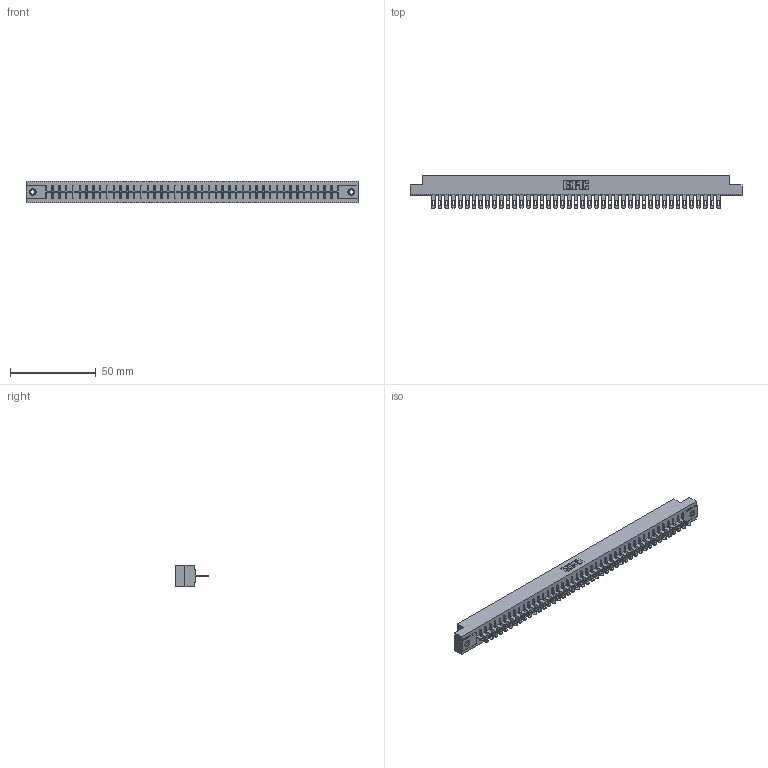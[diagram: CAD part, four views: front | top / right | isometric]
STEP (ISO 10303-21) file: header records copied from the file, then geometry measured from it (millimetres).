
FILE_DESCRIPTION (( 'STEP AP203' ), '1' );
FILE_NAME ('356-043-400-107.STEP', '2020-09-24T01:46:20', ( '' ), ( '' ), 'SwSTEP 2.0', 'SolidWorks 2020', '' );
FILE_SCHEMA (( 'CONFIG_CONTROL_DESIGN' ));
Length unit declared in the file: inch
Products named in the file (4): 345-250-001_345-250-005-103; 306-290-001_100; 306 Part_.156 Dia; 356-043-400-107
Assembly tree (46 placements, depth 2):
  356-043-400-107
    306 Part_.156 Dia
    306-290-001_100  x43
    345-250-001_345-250-005-103  x2
Bounding box: 193.4 x 18.87 x 12.7 mm (x, y, z)
Volume: 21521.9 mm3; surface area: 22895.1 mm2
Topology: 46 solids, 46 shells, 3444 faces, 9697 edges, 6226 vertices
Faces by surface type: plane 2250, cylinder 1006, sphere 172, cone 12, torus 4
Entity records: 41319 total; most frequent: CARTESIAN_POINT 6919, ORIENTED_EDGE 6854, DIRECTION 6831, EDGE_CURVE 3427, LINE 2679, VECTOR 2679, VERTEX_POINT 2164, AXIS2_PLACEMENT_3D 2076
